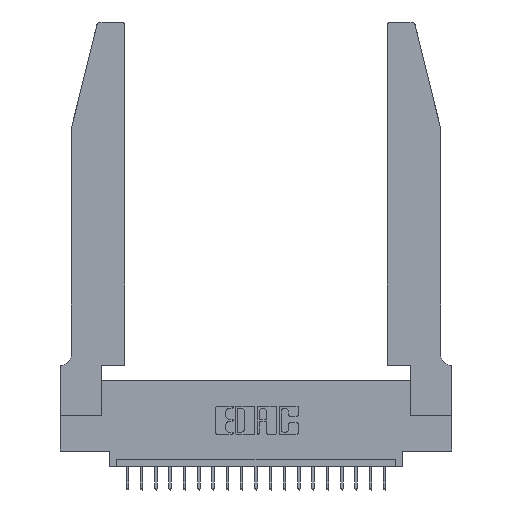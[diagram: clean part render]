
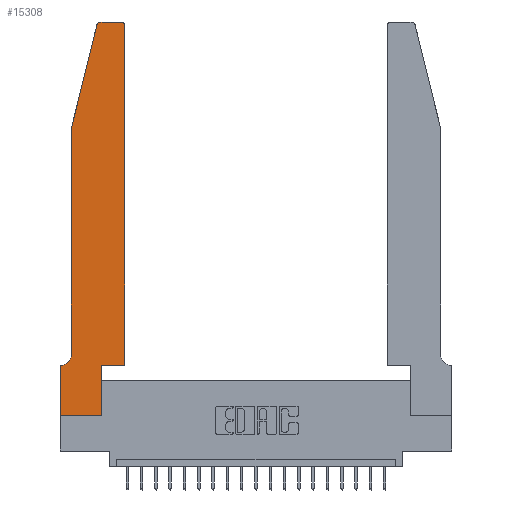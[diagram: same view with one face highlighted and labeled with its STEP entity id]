
A CAD part, top view. The second image highlights one B-rep face of the part: STEP entity #15308.
In plain terms, the highlighted planar face has unit normal (0, 0, 1).
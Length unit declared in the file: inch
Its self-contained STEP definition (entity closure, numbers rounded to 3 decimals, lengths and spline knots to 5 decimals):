
#255 = ORIENTED_EDGE ( 'NONE', *, *, #8281, .T. ) ;
#537 = ORIENTED_EDGE ( 'NONE', *, *, #11519, .T. ) ;
#603 = AXIS2_PLACEMENT_3D ( 'NONE', #5752, #4273, #19553 ) ;
#625 = EDGE_CURVE ( 'NONE', #21234, #16144, #9159, .T. ) ;
#626 = CARTESIAN_POINT ( 'NONE',  ( 0.4505, 0.35, 0.37 ) ) ;
#2044 = VECTOR ( 'NONE', #12556, 39.37008 ) ;
#2102 = DIRECTION ( 'NONE',  ( -1., 0., 0. ) ) ;
#2350 = EDGE_CURVE ( 'NONE', #6574, #18049, #8787, .T. ) ;
#2394 = AXIS2_PLACEMENT_3D ( 'NONE', #6376, #11586, #3141 ) ;
#2465 = CARTESIAN_POINT ( 'NONE',  ( 0.2865, 0.35, 0.37 ) ) ;
#3048 = DIRECTION ( 'NONE',  ( -1., 0., 0. ) ) ;
#3141 = DIRECTION ( 'NONE',  ( 1., 0., 0. ) ) ;
#3269 = LINE ( 'NONE', #626, #12433 ) ;
#3271 = DIRECTION ( 'NONE',  ( 0., -1., 0. ) ) ;
#3956 = CARTESIAN_POINT ( 'NONE',  ( 0.4205, 2.72, 0.37 ) ) ;
#3960 = LINE ( 'NONE', #20128, #7976 ) ;
#4273 = DIRECTION ( 'NONE',  ( 0., 0., -1. ) ) ;
#4914 = EDGE_CURVE ( 'NONE', #5715, #13864, #20489, .T. ) ;
#5562 = LINE ( 'NONE', #10940, #17406 ) ;
#5686 = ORIENTED_EDGE ( 'NONE', *, *, #16176, .T. ) ;
#5715 = VERTEX_POINT ( 'NONE', #9367 ) ;
#5752 = CARTESIAN_POINT ( 'NONE',  ( 0.0055, 0.42, 0.37 ) ) ;
#5996 = VERTEX_POINT ( 'NONE', #14664 ) ;
#6170 = CARTESIAN_POINT ( 'NONE',  ( 0.0755, 2., 0.37 ) ) ;
#6257 = DIRECTION ( 'NONE',  ( 1., 0., 0. ) ) ;
#6374 = CARTESIAN_POINT ( 'NONE',  ( 0.0755, 2., 0.37 ) ) ;
#6376 = CARTESIAN_POINT ( 'NONE',  ( 0.284, 2.72, 0.37 ) ) ;
#6574 = VERTEX_POINT ( 'NONE', #9694 ) ;
#6875 = VECTOR ( 'NONE', #16181, 39.37008 ) ;
#6904 = VERTEX_POINT ( 'NONE', #6374 ) ;
#7475 = CARTESIAN_POINT ( 'NONE',  ( 0.4505, 0.35, 0.37 ) ) ;
#7976 = VECTOR ( 'NONE', #15356, 39.37008 ) ;
#8071 = EDGE_CURVE ( 'NONE', #6904, #21234, #3960, .T. ) ;
#8281 = EDGE_CURVE ( 'NONE', #14964, #5996, #13348, .T. ) ;
#8698 = CARTESIAN_POINT ( 'NONE',  ( 0., 0.35, 0.37 ) ) ;
#8787 = LINE ( 'NONE', #10760, #2044 ) ;
#9159 = CIRCLE ( 'NONE', #603, 0.07 ) ;
#9267 = VERTEX_POINT ( 'NONE', #10456 ) ;
#9281 = DIRECTION ( 'NONE',  ( 0., 1., 0. ) ) ;
#9367 = CARTESIAN_POINT ( 'NONE',  ( 0.284, 2.75, 0.37 ) ) ;
#9694 = CARTESIAN_POINT ( 'NONE',  ( 0., 0., 0.37 ) ) ;
#10050 = FACE_OUTER_BOUND ( 'NONE', #15547, .T. ) ;
#10063 = LINE ( 'NONE', #17298, #21104 ) ;
#10181 = DIRECTION ( 'NONE',  ( 1., 0., 0. ) ) ;
#10456 = CARTESIAN_POINT ( 'NONE',  ( 0.4205, 2.75, 0.37 ) ) ;
#10760 = CARTESIAN_POINT ( 'NONE',  ( 0., 0., 0.37 ) ) ;
#10910 = EDGE_CURVE ( 'NONE', #13864, #6904, #20744, .T. ) ;
#10940 = CARTESIAN_POINT ( 'NONE',  ( 0.2865, 0.35, 0.37 ) ) ;
#11329 = DIRECTION ( 'NONE',  ( 1., 0., 0. ) ) ;
#11519 = EDGE_CURVE ( 'NONE', #9267, #5715, #15028, .T. ) ;
#11586 = DIRECTION ( 'NONE',  ( 0., 0., 1. ) ) ;
#11914 = ORIENTED_EDGE ( 'NONE', *, *, #4914, .T. ) ;
#12388 = VECTOR ( 'NONE', #16531, 39.37008 ) ;
#12433 = VECTOR ( 'NONE', #11329, 39.37008 ) ;
#12556 = DIRECTION ( 'NONE',  ( 1., 0., 0. ) ) ;
#13348 = LINE ( 'NONE', #7475, #6875 ) ;
#13469 = DIRECTION ( 'NONE',  ( 0., 0., 1. ) ) ;
#13543 = CARTESIAN_POINT ( 'NONE',  ( 0., 0.35, 0.37 ) ) ;
#13567 = CARTESIAN_POINT ( 'NONE',  ( 0., 0., 0.37 ) ) ;
#13864 = VERTEX_POINT ( 'NONE', #20594 ) ;
#13950 = EDGE_CURVE ( 'NONE', #15906, #6574, #15217, .T. ) ;
#14340 = VERTEX_POINT ( 'NONE', #2465 ) ;
#14373 = ORIENTED_EDGE ( 'NONE', *, *, #15049, .T. ) ;
#14664 = CARTESIAN_POINT ( 'NONE',  ( 0.4505, 2.72, 0.37 ) ) ;
#14730 = ORIENTED_EDGE ( 'NONE', *, *, #625, .T. ) ;
#14964 = VERTEX_POINT ( 'NONE', #22075 ) ;
#15028 = LINE ( 'NONE', #20002, #21260 ) ;
#15042 = EDGE_CURVE ( 'NONE', #16144, #15906, #10063, .T. ) ;
#15049 = EDGE_CURVE ( 'NONE', #5996, #9267, #20298, .T. ) ;
#15060 = PLANE ( 'NONE',  #15316 ) ;
#15217 = LINE ( 'NONE', #13567, #19268 ) ;
#15277 = DIRECTION ( 'NONE',  ( 0., 0., 1. ) ) ;
#15301 = ORIENTED_EDGE ( 'NONE', *, *, #10910, .T. ) ;
#15308 = ADVANCED_FACE ( 'NONE', ( #10050 ), #15060, .T. ) ;
#15316 = AXIS2_PLACEMENT_3D ( 'NONE', #13543, #15277, #10181 ) ;
#15356 = DIRECTION ( 'NONE',  ( 0., -1., 0. ) ) ;
#15547 = EDGE_LOOP ( 'NONE', ( #537, #11914, #15301, #20224, #14730, #20969, #19714, #17717, #16794, #5686, #255, #14373 ) ) ;
#15906 = VERTEX_POINT ( 'NONE', #8698 ) ;
#16144 = VERTEX_POINT ( 'NONE', #18699 ) ;
#16176 = EDGE_CURVE ( 'NONE', #14340, #14964, #3269, .T. ) ;
#16181 = DIRECTION ( 'NONE',  ( 0., 1., 0. ) ) ;
#16531 = DIRECTION ( 'NONE',  ( -0.239, -0.971, 0. ) ) ;
#16794 = ORIENTED_EDGE ( 'NONE', *, *, #20614, .T. ) ;
#17298 = CARTESIAN_POINT ( 'NONE',  ( 0.0755, 0.35, 0.37 ) ) ;
#17406 = VECTOR ( 'NONE', #9281, 39.37008 ) ;
#17717 = ORIENTED_EDGE ( 'NONE', *, *, #2350, .T. ) ;
#18049 = VERTEX_POINT ( 'NONE', #19977 ) ;
#18699 = CARTESIAN_POINT ( 'NONE',  ( 0.0055, 0.35, 0.37 ) ) ;
#19268 = VECTOR ( 'NONE', #3271, 39.37008 ) ;
#19326 = CARTESIAN_POINT ( 'NONE',  ( 0.0755, 0.42, 0.37 ) ) ;
#19553 = DIRECTION ( 'NONE',  ( -1., 0., 0. ) ) ;
#19714 = ORIENTED_EDGE ( 'NONE', *, *, #13950, .T. ) ;
#19977 = CARTESIAN_POINT ( 'NONE',  ( 0.2865, 0., 0.37 ) ) ;
#20002 = CARTESIAN_POINT ( 'NONE',  ( 0.2605, 2.75, 0.37 ) ) ;
#20128 = CARTESIAN_POINT ( 'NONE',  ( 0.0755, 2., 0.37 ) ) ;
#20224 = ORIENTED_EDGE ( 'NONE', *, *, #8071, .T. ) ;
#20298 = CIRCLE ( 'NONE', #21867, 0.03 ) ;
#20489 = CIRCLE ( 'NONE', #2394, 0.03 ) ;
#20594 = CARTESIAN_POINT ( 'NONE',  ( 0.25487, 2.72718, 0.37 ) ) ;
#20614 = EDGE_CURVE ( 'NONE', #18049, #14340, #5562, .T. ) ;
#20744 = LINE ( 'NONE', #6170, #12388 ) ;
#20969 = ORIENTED_EDGE ( 'NONE', *, *, #15042, .T. ) ;
#21104 = VECTOR ( 'NONE', #2102, 39.37008 ) ;
#21234 = VERTEX_POINT ( 'NONE', #19326 ) ;
#21260 = VECTOR ( 'NONE', #3048, 39.37008 ) ;
#21867 = AXIS2_PLACEMENT_3D ( 'NONE', #3956, #13469, #6257 ) ;
#22075 = CARTESIAN_POINT ( 'NONE',  ( 0.4505, 0.35, 0.37 ) ) ;
